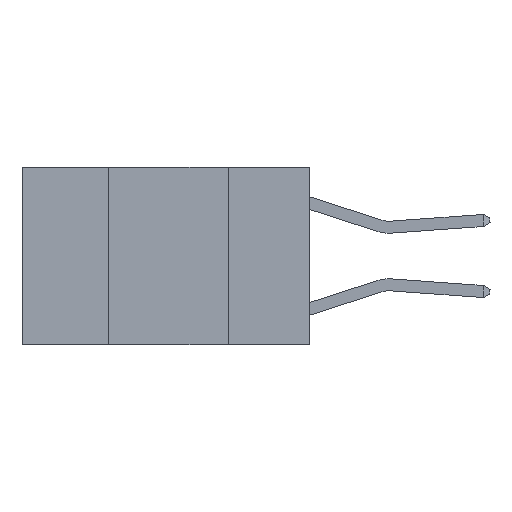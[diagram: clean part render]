
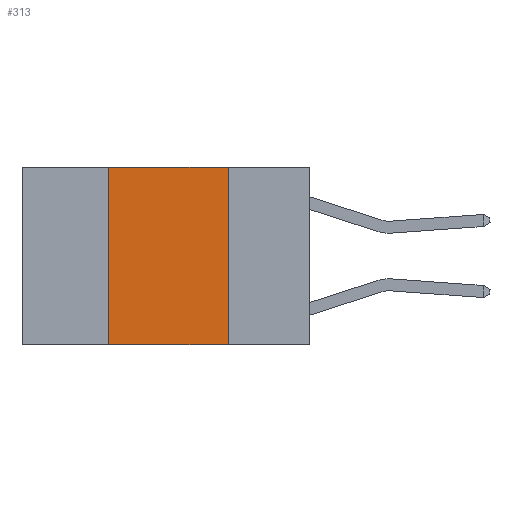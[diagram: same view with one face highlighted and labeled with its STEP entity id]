
A CAD part, left-side view. The second image highlights one B-rep face of the part: STEP entity #313.
In plain terms, the highlighted planar face has unit normal (-1, 0, 0).
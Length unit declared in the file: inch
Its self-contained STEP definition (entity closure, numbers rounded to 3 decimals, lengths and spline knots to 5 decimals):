
#10 = EDGE_CURVE ( 'NONE', #8269, #4436, #7652, .T. ) ;
#205 = VECTOR ( 'NONE', #12924, 39.37008 ) ;
#259 = CARTESIAN_POINT ( 'NONE',  ( 0., 0.17, -0.37 ) ) ;
#313 = ADVANCED_FACE ( 'NONE', ( #9241 ), #22807, .F. ) ;
#1442 = VERTEX_POINT ( 'NONE', #5576 ) ;
#1502 = VECTOR ( 'NONE', #14021, 39.37008 ) ;
#2318 = EDGE_LOOP ( 'NONE', ( #9116, #28389, #28449, #12807 ) ) ;
#3711 = EDGE_CURVE ( 'NONE', #1442, #6685, #14697, .T. ) ;
#3877 = CARTESIAN_POINT ( 'NONE',  ( 0., 0.6, -0.37 ) ) ;
#4436 = VERTEX_POINT ( 'NONE', #259 ) ;
#5104 = VECTOR ( 'NONE', #8324, 39.37008 ) ;
#5576 = CARTESIAN_POINT ( 'NONE',  ( 0., 0.42, -0.37 ) ) ;
#6685 = VERTEX_POINT ( 'NONE', #14239 ) ;
#7083 = DIRECTION ( 'NONE',  ( 0., 0., -1. ) ) ;
#7652 = LINE ( 'NONE', #9746, #22032 ) ;
#8269 = VERTEX_POINT ( 'NONE', #14444 ) ;
#8324 = DIRECTION ( 'NONE',  ( 0., 0., 1. ) ) ;
#9116 = ORIENTED_EDGE ( 'NONE', *, *, #10, .F. ) ;
#9241 = FACE_OUTER_BOUND ( 'NONE', #2318, .T. ) ;
#9746 = CARTESIAN_POINT ( 'NONE',  ( 0., 0.17, 0. ) ) ;
#11521 = CARTESIAN_POINT ( 'NONE',  ( 0., 0.6, 0. ) ) ;
#12807 = ORIENTED_EDGE ( 'NONE', *, *, #18940, .T. ) ;
#12924 = DIRECTION ( 'NONE',  ( 0., -1., 0. ) ) ;
#14021 = DIRECTION ( 'NONE',  ( 0., -1., 0. ) ) ;
#14239 = CARTESIAN_POINT ( 'NONE',  ( 0., 0.42, 0. ) ) ;
#14444 = CARTESIAN_POINT ( 'NONE',  ( 0., 0.17, 0. ) ) ;
#14697 = LINE ( 'NONE', #19116, #5104 ) ;
#15798 = EDGE_CURVE ( 'NONE', #6685, #8269, #22863, .T. ) ;
#18940 = EDGE_CURVE ( 'NONE', #1442, #4436, #26359, .T. ) ;
#19116 = CARTESIAN_POINT ( 'NONE',  ( 0., 0.42, 0. ) ) ;
#22032 = VECTOR ( 'NONE', #7083, 39.37008 ) ;
#22519 = CARTESIAN_POINT ( 'NONE',  ( 0., 0.6, 0. ) ) ;
#22670 = DIRECTION ( 'NONE',  ( 0., 0., -1. ) ) ;
#22807 = PLANE ( 'NONE',  #24105 ) ;
#22863 = LINE ( 'NONE', #11521, #1502 ) ;
#24105 = AXIS2_PLACEMENT_3D ( 'NONE', #22519, #29166, #22670 ) ;
#26359 = LINE ( 'NONE', #3877, #205 ) ;
#28389 = ORIENTED_EDGE ( 'NONE', *, *, #15798, .F. ) ;
#28449 = ORIENTED_EDGE ( 'NONE', *, *, #3711, .F. ) ;
#29166 = DIRECTION ( 'NONE',  ( 1., 0., 0. ) ) ;
